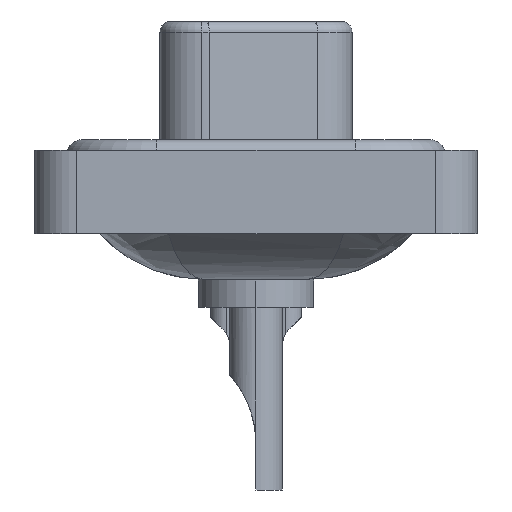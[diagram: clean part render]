
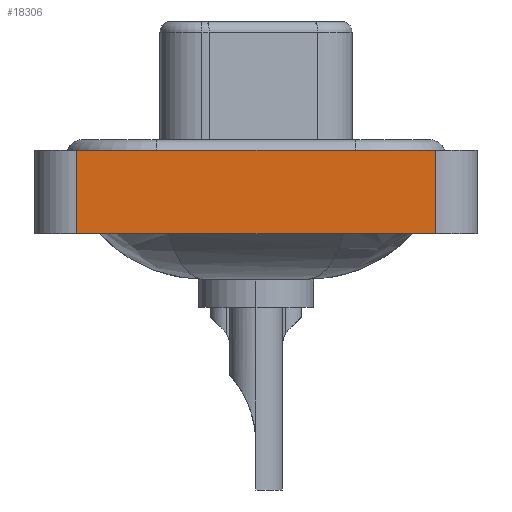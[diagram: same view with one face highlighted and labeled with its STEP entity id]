
A CAD part, left-side view. The second image highlights one B-rep face of the part: STEP entity #18306.
In plain terms, the highlighted planar face has unit normal (-1, 0, 0).
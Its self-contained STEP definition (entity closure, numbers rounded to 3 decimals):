
#1578 = DIRECTION ( 'NONE',  ( -1., 0., 0. ) ) ;
#1827 = LINE ( 'NONE', #9030, #3246 ) ;
#2055 = ORIENTED_EDGE ( 'NONE', *, *, #11242, .F. ) ;
#2640 = ORIENTED_EDGE ( 'NONE', *, *, #17219, .F. ) ;
#3246 = VECTOR ( 'NONE', #3356, 1000. ) ;
#3347 = VERTEX_POINT ( 'NONE', #9380 ) ;
#3356 = DIRECTION ( 'NONE',  ( 0., -1., 0. ) ) ;
#4554 = VECTOR ( 'NONE', #12721, 1000. ) ;
#5172 = EDGE_LOOP ( 'NONE', ( #13011, #2640, #2055, #17839 ) ) ;
#6457 = CARTESIAN_POINT ( 'NONE',  ( -7.35, 8.55, -3.6 ) ) ;
#6542 = PLANE ( 'NONE',  #22807 ) ;
#7350 = DIRECTION ( 'NONE',  ( 0., 0., 1. ) ) ;
#8740 = CARTESIAN_POINT ( 'NONE',  ( -7.35, -8.55, -3.6 ) ) ;
#9030 = CARTESIAN_POINT ( 'NONE',  ( -7.35, -8.55, -3.6 ) ) ;
#9380 = CARTESIAN_POINT ( 'NONE',  ( -7.35, -8.55, 0.4 ) ) ;
#9907 = VERTEX_POINT ( 'NONE', #6457 ) ;
#10094 = FACE_OUTER_BOUND ( 'NONE', #5172, .T. ) ;
#10326 = DIRECTION ( 'NONE',  ( 0., 0., 1. ) ) ;
#10491 = CARTESIAN_POINT ( 'NONE',  ( -7.35, 8.55, -3.6 ) ) ;
#11242 = EDGE_CURVE ( 'NONE', #9907, #11249, #21338, .T. ) ;
#11249 = VERTEX_POINT ( 'NONE', #21101 ) ;
#12658 = EDGE_CURVE ( 'NONE', #20792, #3347, #16167, .T. ) ;
#12721 = DIRECTION ( 'NONE',  ( 0., -1., 0. ) ) ;
#13011 = ORIENTED_EDGE ( 'NONE', *, *, #12658, .T. ) ;
#13692 = DIRECTION ( 'NONE',  ( 0., 0., 1. ) ) ;
#13743 = CARTESIAN_POINT ( 'NONE',  ( -7.35, -8.55, -3.6 ) ) ;
#16167 = LINE ( 'NONE', #18204, #22664 ) ;
#16234 = LINE ( 'NONE', #21676, #4554 ) ;
#17219 = EDGE_CURVE ( 'NONE', #11249, #3347, #16234, .T. ) ;
#17839 = ORIENTED_EDGE ( 'NONE', *, *, #19548, .T. ) ;
#18204 = CARTESIAN_POINT ( 'NONE',  ( -7.35, -8.55, -3.6 ) ) ;
#18306 = ADVANCED_FACE ( 'NONE', ( #10094 ), #6542, .T. ) ;
#19548 = EDGE_CURVE ( 'NONE', #9907, #20792, #1827, .T. ) ;
#20792 = VERTEX_POINT ( 'NONE', #8740 ) ;
#21101 = CARTESIAN_POINT ( 'NONE',  ( -7.35, 8.55, 0.4 ) ) ;
#21338 = LINE ( 'NONE', #10491, #22708 ) ;
#21676 = CARTESIAN_POINT ( 'NONE',  ( -7.35, -8.55, 0.4 ) ) ;
#22664 = VECTOR ( 'NONE', #7350, 1000. ) ;
#22708 = VECTOR ( 'NONE', #13692, 1000. ) ;
#22807 = AXIS2_PLACEMENT_3D ( 'NONE', #13743, #1578, #10326 ) ;
